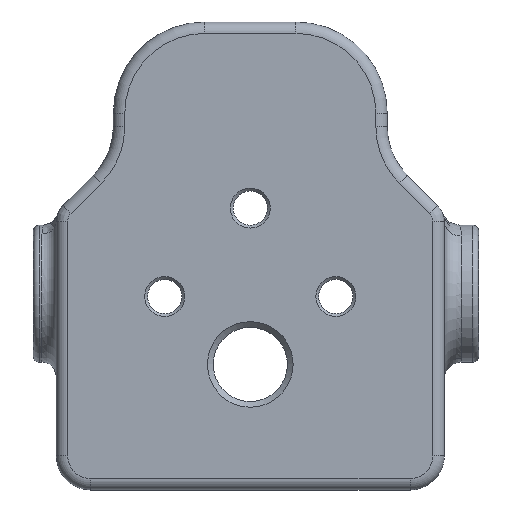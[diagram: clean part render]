
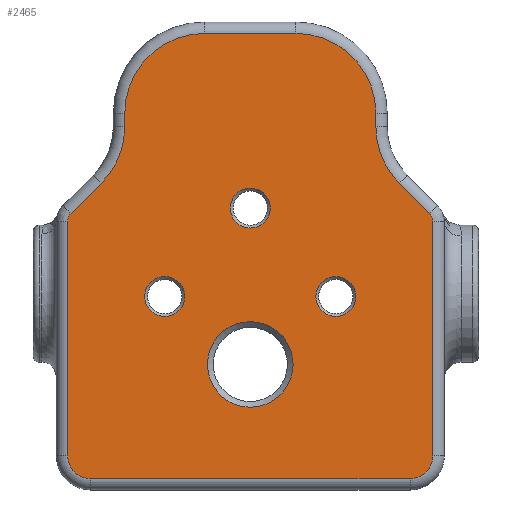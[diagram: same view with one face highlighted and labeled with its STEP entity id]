
A CAD part, left-side view. The second image highlights one B-rep face of the part: STEP entity #2465.
In plain terms, the highlighted planar face has unit normal (-1, 0, 0).
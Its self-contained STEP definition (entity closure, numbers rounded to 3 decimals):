
#41=LINE('',#3982,#194);
#42=LINE('',#3986,#195);
#43=LINE('',#3990,#196);
#44=LINE('',#3994,#197);
#45=LINE('',#3998,#198);
#46=LINE('',#4002,#199);
#47=LINE('',#4006,#200);
#48=LINE('',#4010,#201);
#194=VECTOR('',#3038,10.);
#195=VECTOR('',#3041,10.);
#196=VECTOR('',#3044,10.);
#197=VECTOR('',#3047,10.);
#198=VECTOR('',#3050,10.);
#199=VECTOR('',#3053,10.);
#200=VECTOR('',#3056,10.);
#201=VECTOR('',#3059,10.);
#387=FACE_BOUND('',#649,.T.);
#388=FACE_BOUND('',#650,.T.);
#389=FACE_BOUND('',#651,.T.);
#390=FACE_BOUND('',#652,.T.);
#407=PLANE('',#2665);
#488=FACE_OUTER_BOUND('',#648,.T.);
#648=EDGE_LOOP('',(#1719,#1720,#1721,#1722,#1723,#1724,#1725,#1726,#1727,
#1728,#1729,#1730,#1731,#1732,#1733,#1734));
#649=EDGE_LOOP('',(#1735));
#650=EDGE_LOOP('',(#1736));
#651=EDGE_LOOP('',(#1737));
#652=EDGE_LOOP('',(#1738));
#841=CIRCLE('',#2662,1.75);
#843=CIRCLE('',#2666,1.);
#844=CIRCLE('',#2667,2.);
#845=CIRCLE('',#2668,2.);
#846=CIRCLE('',#2669,1.);
#847=CIRCLE('',#2670,7.);
#848=CIRCLE('',#2671,7.);
#849=CIRCLE('',#2672,7.);
#850=CIRCLE('',#2673,7.);
#851=CIRCLE('',#2674,1.75);
#852=CIRCLE('',#2675,3.75);
#853=CIRCLE('',#2676,1.75);
#1070=VERTEX_POINT('',#3972);
#1072=VERTEX_POINT('',#3980);
#1073=VERTEX_POINT('',#3981);
#1074=VERTEX_POINT('',#3983);
#1075=VERTEX_POINT('',#3985);
#1076=VERTEX_POINT('',#3987);
#1077=VERTEX_POINT('',#3989);
#1078=VERTEX_POINT('',#3991);
#1079=VERTEX_POINT('',#3993);
#1080=VERTEX_POINT('',#3995);
#1081=VERTEX_POINT('',#3997);
#1082=VERTEX_POINT('',#3999);
#1083=VERTEX_POINT('',#4001);
#1084=VERTEX_POINT('',#4003);
#1085=VERTEX_POINT('',#4005);
#1086=VERTEX_POINT('',#4007);
#1087=VERTEX_POINT('',#4009);
#1088=VERTEX_POINT('',#4012);
#1089=VERTEX_POINT('',#4014);
#1090=VERTEX_POINT('',#4016);
#1311=EDGE_CURVE('',#1070,#1070,#841,.T.);
#1314=EDGE_CURVE('',#1072,#1073,#41,.T.);
#1315=EDGE_CURVE('',#1074,#1072,#843,.T.);
#1316=EDGE_CURVE('',#1075,#1074,#42,.T.);
#1317=EDGE_CURVE('',#1076,#1075,#844,.T.);
#1318=EDGE_CURVE('',#1077,#1076,#43,.T.);
#1319=EDGE_CURVE('',#1078,#1077,#845,.T.);
#1320=EDGE_CURVE('',#1079,#1078,#44,.T.);
#1321=EDGE_CURVE('',#1080,#1079,#846,.T.);
#1322=EDGE_CURVE('',#1081,#1080,#45,.T.);
#1323=EDGE_CURVE('',#1082,#1081,#847,.T.);
#1324=EDGE_CURVE('',#1083,#1082,#46,.T.);
#1325=EDGE_CURVE('',#1084,#1083,#848,.T.);
#1326=EDGE_CURVE('',#1085,#1084,#47,.T.);
#1327=EDGE_CURVE('',#1086,#1085,#849,.T.);
#1328=EDGE_CURVE('',#1087,#1086,#48,.T.);
#1329=EDGE_CURVE('',#1073,#1087,#850,.T.);
#1330=EDGE_CURVE('',#1088,#1088,#851,.T.);
#1331=EDGE_CURVE('',#1089,#1089,#852,.T.);
#1332=EDGE_CURVE('',#1090,#1090,#853,.T.);
#1719=ORIENTED_EDGE('',*,*,#1314,.F.);
#1720=ORIENTED_EDGE('',*,*,#1315,.F.);
#1721=ORIENTED_EDGE('',*,*,#1316,.F.);
#1722=ORIENTED_EDGE('',*,*,#1317,.F.);
#1723=ORIENTED_EDGE('',*,*,#1318,.F.);
#1724=ORIENTED_EDGE('',*,*,#1319,.F.);
#1725=ORIENTED_EDGE('',*,*,#1320,.F.);
#1726=ORIENTED_EDGE('',*,*,#1321,.F.);
#1727=ORIENTED_EDGE('',*,*,#1322,.F.);
#1728=ORIENTED_EDGE('',*,*,#1323,.F.);
#1729=ORIENTED_EDGE('',*,*,#1324,.F.);
#1730=ORIENTED_EDGE('',*,*,#1325,.F.);
#1731=ORIENTED_EDGE('',*,*,#1326,.F.);
#1732=ORIENTED_EDGE('',*,*,#1327,.F.);
#1733=ORIENTED_EDGE('',*,*,#1328,.F.);
#1734=ORIENTED_EDGE('',*,*,#1329,.F.);
#1735=ORIENTED_EDGE('',*,*,#1330,.F.);
#1736=ORIENTED_EDGE('',*,*,#1331,.F.);
#1737=ORIENTED_EDGE('',*,*,#1332,.F.);
#1738=ORIENTED_EDGE('',*,*,#1311,.F.);
#2465=ADVANCED_FACE('',(#488,#387,#388,#389,#390),#407,.F.);
#2662=AXIS2_PLACEMENT_3D('',#3974,#3029,#3030);
#2665=AXIS2_PLACEMENT_3D('',#3979,#3036,#3037);
#2666=AXIS2_PLACEMENT_3D('',#3984,#3039,#3040);
#2667=AXIS2_PLACEMENT_3D('',#3988,#3042,#3043);
#2668=AXIS2_PLACEMENT_3D('',#3992,#3045,#3046);
#2669=AXIS2_PLACEMENT_3D('',#3996,#3048,#3049);
#2670=AXIS2_PLACEMENT_3D('',#4000,#3051,#3052);
#2671=AXIS2_PLACEMENT_3D('',#4004,#3054,#3055);
#2672=AXIS2_PLACEMENT_3D('',#4008,#3057,#3058);
#2673=AXIS2_PLACEMENT_3D('',#4011,#3060,#3061);
#2674=AXIS2_PLACEMENT_3D('',#4013,#3062,#3063);
#2675=AXIS2_PLACEMENT_3D('',#4015,#3064,#3065);
#2676=AXIS2_PLACEMENT_3D('',#4017,#3066,#3067);
#3029=DIRECTION('center_axis',(-1.,0.,0.));
#3030=DIRECTION('ref_axis',(0.,0.,
-1.));
#3036=DIRECTION('center_axis',(1.,0.,0.));
#3037=DIRECTION('ref_axis',(0.,0.,-1.));
#3038=DIRECTION('',(0.,-0.707,0.707));
#3039=DIRECTION('center_axis',(1.,0.,0.));
#3040=DIRECTION('ref_axis',(0.,0.924,0.383));
#3041=DIRECTION('',(0.,0.,1.));
#3042=DIRECTION('center_axis',(1.,0.,0.));
#3043=DIRECTION('ref_axis',(0.,0.707,-0.707));
#3044=DIRECTION('',(0.,1.,0.));
#3045=DIRECTION('center_axis',(1.,0.,0.));
#3046=DIRECTION('ref_axis',(0.,-0.707,-0.707));
#3047=DIRECTION('',(0.,0.,-1.));
#3048=DIRECTION('center_axis',(1.,0.,0.));
#3049=DIRECTION('ref_axis',(0.,-0.924,0.383));
#3050=DIRECTION('',(0.,-0.707,-0.707));
#3051=DIRECTION('center_axis',(-1.,0.,0.));
#3052=DIRECTION('ref_axis',(0.,0.924,-0.383));
#3053=DIRECTION('',(0.,0.,-1.));
#3054=DIRECTION('center_axis',(1.,0.,0.));
#3055=DIRECTION('ref_axis',(0.,-0.707,0.707));
#3056=DIRECTION('',(0.,-1.,0.));
#3057=DIRECTION('center_axis',(1.,0.,0.));
#3058=DIRECTION('ref_axis',(0.,0.707,0.707));
#3059=DIRECTION('',(0.,0.,1.));
#3060=DIRECTION('center_axis',(-1.,0.,0.));
#3061=DIRECTION('ref_axis',(0.,-0.924,-0.383));
#3062=DIRECTION('center_axis',(-1.,0.,0.));
#3063=DIRECTION('ref_axis',(0.,0.,
-1.));
#3064=DIRECTION('center_axis',(-1.,0.,0.));
#3065=DIRECTION('ref_axis',(0.,0.,
-1.));
#3066=DIRECTION('center_axis',(-1.,0.,0.));
#3067=DIRECTION('ref_axis',(0.,0.,
-1.));
#3972=CARTESIAN_POINT('',(130.981,0.,-85.553));
#3974=CARTESIAN_POINT('Origin',(130.981,0.,
-87.303));
#3979=CARTESIAN_POINT('Origin',(130.981,0.,
-91.5));
#3980=CARTESIAN_POINT('',(130.981,15.707,-87.778));
#3981=CARTESIAN_POINT('',(130.981,13.05,-85.121));
#3982=CARTESIAN_POINT('',(130.981,13.004,-85.075));
#3983=CARTESIAN_POINT('',(130.981,16.,-88.485));
#3984=CARTESIAN_POINT('Origin',(130.981,15.,-88.485));
#3985=CARTESIAN_POINT('',(130.981,16.,-109.));
#3986=CARTESIAN_POINT('',(130.981,16.,-101.75));
#3987=CARTESIAN_POINT('',(130.981,14.,-111.));
#3988=CARTESIAN_POINT('Origin',(130.981,14.,-109.));
#3989=CARTESIAN_POINT('',(130.981,-14.,-111.));
#3990=CARTESIAN_POINT('',(130.981,-8.5,-111.));
#3991=CARTESIAN_POINT('',(130.981,-16.,-109.));
#3992=CARTESIAN_POINT('Origin',(130.981,-14.,-109.));
#3993=CARTESIAN_POINT('',(130.981,-16.,-88.485));
#3994=CARTESIAN_POINT('',(130.981,-16.,-89.578));
#3995=CARTESIAN_POINT('',(130.981,-15.707,-87.778));
#3996=CARTESIAN_POINT('Origin',(130.981,-15.,-88.485));
#3997=CARTESIAN_POINT('',(130.981,-13.05,-85.121));
#3998=CARTESIAN_POINT('',(130.981,-11.382,-83.453));
#3999=CARTESIAN_POINT('',(130.981,-11.,-80.172));
#4000=CARTESIAN_POINT('Origin',(130.981,-18.,-80.172));
#4001=CARTESIAN_POINT('',(130.981,-11.,-79.));
#4002=CARTESIAN_POINT('',(130.981,-11.,-85.25));
#4003=CARTESIAN_POINT('',(130.981,-4.,-72.));
#4004=CARTESIAN_POINT('Origin',(130.981,-4.,-79.));
#4005=CARTESIAN_POINT('',(130.981,4.,-72.));
#4006=CARTESIAN_POINT('',(130.981,2.,-72.));
#4007=CARTESIAN_POINT('',(130.981,11.,-79.));
#4008=CARTESIAN_POINT('Origin',(130.981,4.,-79.));
#4009=CARTESIAN_POINT('',(130.981,11.,-80.172));
#4010=CARTESIAN_POINT('',(130.981,11.,-85.836));
#4011=CARTESIAN_POINT('Origin',(130.981,18.,-80.172));
#4012=CARTESIAN_POINT('',(130.981,7.496,-93.303));
#4013=CARTESIAN_POINT('Origin',(130.981,7.496,-95.053));
#4014=CARTESIAN_POINT('',(130.981,0.,-97.25));
#4015=CARTESIAN_POINT('Origin',(130.981,0.,-101.));
#4016=CARTESIAN_POINT('',(130.981,-7.496,-93.303));
#4017=CARTESIAN_POINT('Origin',(130.981,-7.496,-95.053));
